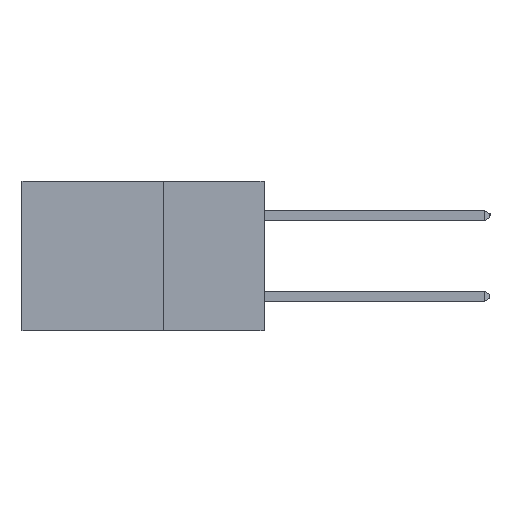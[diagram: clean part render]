
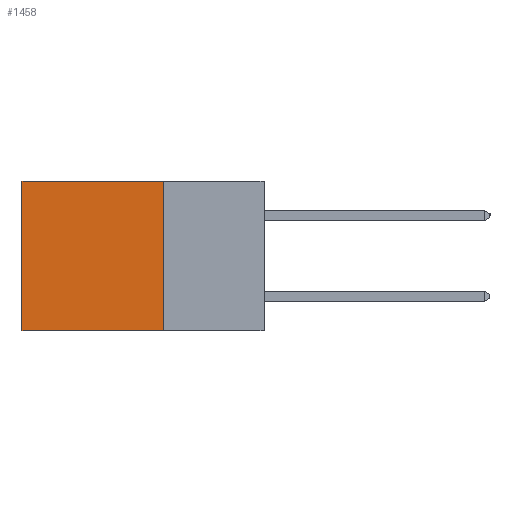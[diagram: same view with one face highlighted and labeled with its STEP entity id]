
A CAD part, left-side view. The second image highlights one B-rep face of the part: STEP entity #1458.
In plain terms, the highlighted planar face has unit normal (-1, 0, 0).
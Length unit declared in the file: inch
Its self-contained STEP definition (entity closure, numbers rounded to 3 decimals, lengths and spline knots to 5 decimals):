
#387 = CARTESIAN_POINT ( 'NONE',  ( 0.2615, 0.25, 0. ) ) ;
#958 = CARTESIAN_POINT ( 'NONE',  ( 0.2615, 0.6, -0.37 ) ) ;
#1458 = ADVANCED_FACE ( 'NONE', ( #10134 ), #9895, .F. ) ;
#2082 = LINE ( 'NONE', #9408, #12161 ) ;
#2719 = ORIENTED_EDGE ( 'NONE', *, *, #9158, .F. ) ;
#2745 = ORIENTED_EDGE ( 'NONE', *, *, #20138, .T. ) ;
#3386 = EDGE_CURVE ( 'NONE', #23619, #17718, #8857, .T. ) ;
#4348 = VERTEX_POINT ( 'NONE', #958 ) ;
#5110 = CARTESIAN_POINT ( 'NONE',  ( 0.2615, 0.25, -0.37 ) ) ;
#5191 = AXIS2_PLACEMENT_3D ( 'NONE', #12039, #10364, #15623 ) ;
#6924 = LINE ( 'NONE', #5110, #15248 ) ;
#7913 = CARTESIAN_POINT ( 'NONE',  ( 0.2615, 0.25, 0. ) ) ;
#8857 = LINE ( 'NONE', #10996, #9111 ) ;
#9023 = ORIENTED_EDGE ( 'NONE', *, *, #10340, .T. ) ;
#9111 = VECTOR ( 'NONE', #21860, 39.37008 ) ;
#9158 = EDGE_CURVE ( 'NONE', #17718, #4348, #6924, .T. ) ;
#9228 = CARTESIAN_POINT ( 'NONE',  ( 0.2615, 0.25, -0.37 ) ) ;
#9408 = CARTESIAN_POINT ( 'NONE',  ( 0.2615, 0.6, -0.37 ) ) ;
#9895 = PLANE ( 'NONE',  #5191 ) ;
#10134 = FACE_OUTER_BOUND ( 'NONE', #12312, .T. ) ;
#10340 = EDGE_CURVE ( 'NONE', #23619, #11378, #17361, .T. ) ;
#10364 = DIRECTION ( 'NONE',  ( 1., 0., 0. ) ) ;
#10996 = CARTESIAN_POINT ( 'NONE',  ( 0.2615, 0.25, -0.37 ) ) ;
#11378 = VERTEX_POINT ( 'NONE', #15691 ) ;
#12039 = CARTESIAN_POINT ( 'NONE',  ( 0.2615, 0.25, -0.37 ) ) ;
#12161 = VECTOR ( 'NONE', #20375, 39.37008 ) ;
#12312 = EDGE_LOOP ( 'NONE', ( #2745, #2719, #15118, #9023 ) ) ;
#15118 = ORIENTED_EDGE ( 'NONE', *, *, #3386, .F. ) ;
#15248 = VECTOR ( 'NONE', #19811, 39.37008 ) ;
#15623 = DIRECTION ( 'NONE',  ( 0., 0., -1. ) ) ;
#15691 = CARTESIAN_POINT ( 'NONE',  ( 0.2615, 0.6, 0. ) ) ;
#16828 = VECTOR ( 'NONE', #20699, 39.37008 ) ;
#17361 = LINE ( 'NONE', #7913, #16828 ) ;
#17718 = VERTEX_POINT ( 'NONE', #9228 ) ;
#19811 = DIRECTION ( 'NONE',  ( 0., 1., 0. ) ) ;
#20138 = EDGE_CURVE ( 'NONE', #11378, #4348, #2082, .T. ) ;
#20375 = DIRECTION ( 'NONE',  ( 0., 0., -1. ) ) ;
#20699 = DIRECTION ( 'NONE',  ( 0., 1., 0. ) ) ;
#21860 = DIRECTION ( 'NONE',  ( 0., 0., -1. ) ) ;
#23619 = VERTEX_POINT ( 'NONE', #387 ) ;
